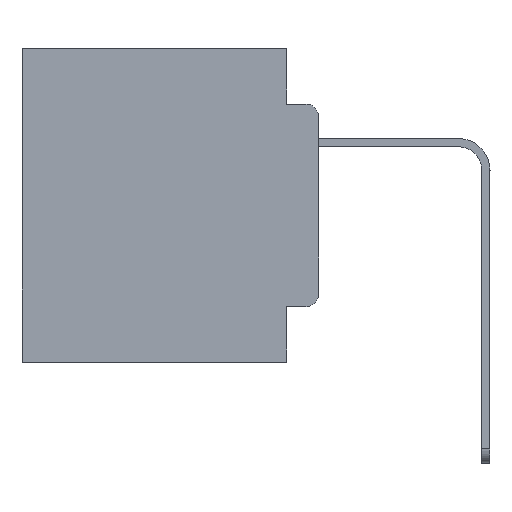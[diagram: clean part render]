
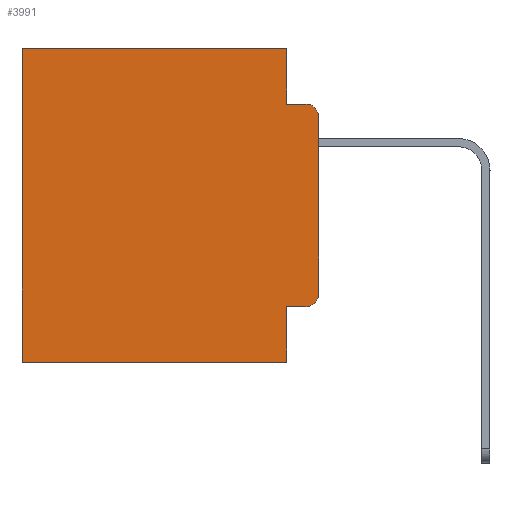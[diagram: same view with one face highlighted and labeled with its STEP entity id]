
A CAD part, left-side view. The second image highlights one B-rep face of the part: STEP entity #3991.
In plain terms, the highlighted planar face has unit normal (-1, 0, 0).
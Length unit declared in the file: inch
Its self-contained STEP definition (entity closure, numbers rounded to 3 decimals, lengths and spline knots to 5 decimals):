
#69 = VECTOR ( 'NONE', #16010, 39.37008 ) ;
#409 = VERTEX_POINT ( 'NONE', #11405 ) ;
#1021 = CARTESIAN_POINT ( 'NONE',  ( 0.298, 0.051, -0.0885 ) ) ;
#1269 = AXIS2_PLACEMENT_3D ( 'NONE', #3280, #13686, #22416 ) ;
#1284 = ORIENTED_EDGE ( 'NONE', *, *, #8661, .T. ) ;
#1514 = EDGE_CURVE ( 'NONE', #25942, #8903, #22471, .T. ) ;
#2083 = ORIENTED_EDGE ( 'NONE', *, *, #16446, .T. ) ;
#2577 = VECTOR ( 'NONE', #11725, 39.37008 ) ;
#3087 = CARTESIAN_POINT ( 'NONE',  ( 0.298, 0.051, -0.4115 ) ) ;
#3113 = VERTEX_POINT ( 'NONE', #1021 ) ;
#3280 = CARTESIAN_POINT ( 'NONE',  ( 0.298, 0.02, -0.1085 ) ) ;
#3991 = ADVANCED_FACE ( 'NONE', ( #6748 ), #7579, .F. ) ;
#4325 = DIRECTION ( 'NONE',  ( 0., 0., -1. ) ) ;
#4702 = CARTESIAN_POINT ( 'NONE',  ( 0.298, 0.473, 0. ) ) ;
#5283 = VECTOR ( 'NONE', #16433, 39.37008 ) ;
#5361 = EDGE_CURVE ( 'NONE', #7975, #8903, #17837, .T. ) ;
#5720 = ORIENTED_EDGE ( 'NONE', *, *, #13808, .F. ) ;
#5870 = CARTESIAN_POINT ( 'NONE',  ( 0.298, 0., 0. ) ) ;
#6065 = DIRECTION ( 'NONE',  ( 1., 0., 0. ) ) ;
#6510 = EDGE_CURVE ( 'NONE', #3113, #409, #10042, .T. ) ;
#6559 = VERTEX_POINT ( 'NONE', #11974 ) ;
#6595 = DIRECTION ( 'NONE',  ( 0., 0., -1. ) ) ;
#6646 = CARTESIAN_POINT ( 'NONE',  ( 0.298, 0.473, -0.5 ) ) ;
#6748 = FACE_OUTER_BOUND ( 'NONE', #11997, .T. ) ;
#6821 = VERTEX_POINT ( 'NONE', #19476 ) ;
#6861 = DIRECTION ( 'NONE',  ( -1., 0., 0. ) ) ;
#7310 = VERTEX_POINT ( 'NONE', #16983 ) ;
#7316 = VERTEX_POINT ( 'NONE', #10704 ) ;
#7371 = LINE ( 'NONE', #3087, #14718 ) ;
#7579 = PLANE ( 'NONE',  #22939 ) ;
#7613 = CARTESIAN_POINT ( 'NONE',  ( 0.298, 0., 0. ) ) ;
#7778 = CARTESIAN_POINT ( 'NONE',  ( 0.298, 0.051, -0.0885 ) ) ;
#7975 = VERTEX_POINT ( 'NONE', #13627 ) ;
#8382 = EDGE_CURVE ( 'NONE', #6559, #7310, #19089, .T. ) ;
#8646 = DIRECTION ( 'NONE',  ( 0., 0., -1. ) ) ;
#8661 = EDGE_CURVE ( 'NONE', #7316, #6559, #7371, .T. ) ;
#8748 = LINE ( 'NONE', #21883, #24197 ) ;
#8903 = VERTEX_POINT ( 'NONE', #6646 ) ;
#9574 = VERTEX_POINT ( 'NONE', #17220 ) ;
#10042 = LINE ( 'NONE', #7778, #25478 ) ;
#10704 = CARTESIAN_POINT ( 'NONE',  ( 0.298, 0.051, -0.4115 ) ) ;
#11405 = CARTESIAN_POINT ( 'NONE',  ( 0.298, 0.02, -0.0885 ) ) ;
#11443 = LINE ( 'NONE', #24176, #69 ) ;
#11599 = DIRECTION ( 'NONE',  ( 0., -1., 0. ) ) ;
#11725 = DIRECTION ( 'NONE',  ( 0., 0., -1. ) ) ;
#11756 = VECTOR ( 'NONE', #27728, 39.37008 ) ;
#11974 = CARTESIAN_POINT ( 'NONE',  ( 0.298, 0.02, -0.4115 ) ) ;
#11997 = EDGE_LOOP ( 'NONE', ( #5720, #15233, #18570, #15097, #2083, #13835, #24226, #22036, #1284, #20382 ) ) ;
#12136 = CARTESIAN_POINT ( 'NONE',  ( 0.298, 0.473, 0. ) ) ;
#13627 = CARTESIAN_POINT ( 'NONE',  ( 0.298, 0.051, -0.5 ) ) ;
#13686 = DIRECTION ( 'NONE',  ( -1., 0., 0. ) ) ;
#13808 = EDGE_CURVE ( 'NONE', #9574, #7310, #21702, .T. ) ;
#13835 = ORIENTED_EDGE ( 'NONE', *, *, #1514, .T. ) ;
#13966 = DIRECTION ( 'NONE',  ( 0., 0., -1. ) ) ;
#13997 = CARTESIAN_POINT ( 'NONE',  ( 0.298, 0., 0. ) ) ;
#14718 = VECTOR ( 'NONE', #11599, 39.37008 ) ;
#15097 = ORIENTED_EDGE ( 'NONE', *, *, #26818, .F. ) ;
#15233 = ORIENTED_EDGE ( 'NONE', *, *, #19634, .T. ) ;
#15423 = VECTOR ( 'NONE', #8646, 39.37008 ) ;
#16010 = DIRECTION ( 'NONE',  ( 0., 0., -1. ) ) ;
#16433 = DIRECTION ( 'NONE',  ( 0., 1., 0. ) ) ;
#16446 = EDGE_CURVE ( 'NONE', #6821, #25942, #19000, .T. ) ;
#16983 = CARTESIAN_POINT ( 'NONE',  ( 0.298, 0., -0.3915 ) ) ;
#17220 = CARTESIAN_POINT ( 'NONE',  ( 0.298, 0., -0.1085 ) ) ;
#17837 = LINE ( 'NONE', #23438, #11756 ) ;
#18570 = ORIENTED_EDGE ( 'NONE', *, *, #6510, .F. ) ;
#19000 = LINE ( 'NONE', #5870, #5283 ) ;
#19089 = CIRCLE ( 'NONE', #24493, 0.02 ) ;
#19476 = CARTESIAN_POINT ( 'NONE',  ( 0.298, 0.051, 0. ) ) ;
#19634 = EDGE_CURVE ( 'NONE', #9574, #409, #25370, .T. ) ;
#20382 = ORIENTED_EDGE ( 'NONE', *, *, #8382, .T. ) ;
#21702 = LINE ( 'NONE', #13997, #2577 ) ;
#21883 = CARTESIAN_POINT ( 'NONE',  ( 0.298, 0.051, 0. ) ) ;
#22036 = ORIENTED_EDGE ( 'NONE', *, *, #25757, .F. ) ;
#22416 = DIRECTION ( 'NONE',  ( 0., 0., -1. ) ) ;
#22471 = LINE ( 'NONE', #4702, #15423 ) ;
#22939 = AXIS2_PLACEMENT_3D ( 'NONE', #7613, #6065, #13966 ) ;
#23438 = CARTESIAN_POINT ( 'NONE',  ( 0.298, 0., -0.5 ) ) ;
#24176 = CARTESIAN_POINT ( 'NONE',  ( 0.298, 0.051, 0. ) ) ;
#24197 = VECTOR ( 'NONE', #6595, 39.37008 ) ;
#24226 = ORIENTED_EDGE ( 'NONE', *, *, #5361, .F. ) ;
#24493 = AXIS2_PLACEMENT_3D ( 'NONE', #25963, #6861, #4325 ) ;
#24917 = DIRECTION ( 'NONE',  ( 0., -1., 0. ) ) ;
#25370 = CIRCLE ( 'NONE', #1269, 0.02 ) ;
#25478 = VECTOR ( 'NONE', #24917, 39.37008 ) ;
#25757 = EDGE_CURVE ( 'NONE', #7316, #7975, #11443, .T. ) ;
#25942 = VERTEX_POINT ( 'NONE', #12136 ) ;
#25963 = CARTESIAN_POINT ( 'NONE',  ( 0.298, 0.02, -0.3915 ) ) ;
#26818 = EDGE_CURVE ( 'NONE', #6821, #3113, #8748, .T. ) ;
#27728 = DIRECTION ( 'NONE',  ( 0., 1., 0. ) ) ;
